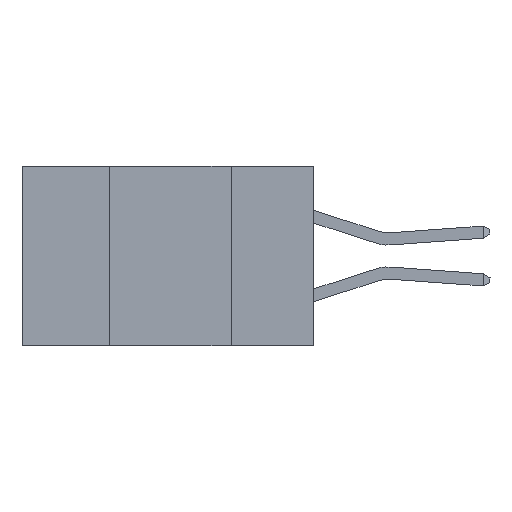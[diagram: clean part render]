
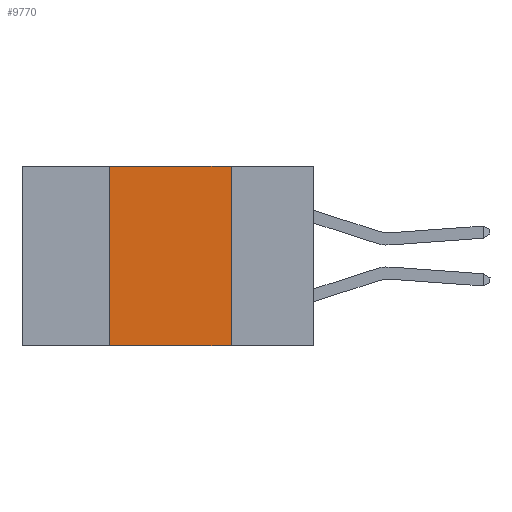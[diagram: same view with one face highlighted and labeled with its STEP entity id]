
A CAD part, left-side view. The second image highlights one B-rep face of the part: STEP entity #9770.
In plain terms, the highlighted planar face has unit normal (-1, 0, 0).
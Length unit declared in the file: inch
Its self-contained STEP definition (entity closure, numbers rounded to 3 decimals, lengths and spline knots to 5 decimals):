
#997 = EDGE_CURVE ( 'NONE', #21251, #8604, #17610, .T. ) ;
#1100 = FACE_OUTER_BOUND ( 'NONE', #4092, .T. ) ;
#1743 = EDGE_CURVE ( 'NONE', #14637, #14149, #7518, .T. ) ;
#2137 = PLANE ( 'NONE',  #11156 ) ;
#4092 = EDGE_LOOP ( 'NONE', ( #19658, #15204, #16624, #13049 ) ) ;
#4861 = CARTESIAN_POINT ( 'NONE',  ( 0., 0.42, 0. ) ) ;
#5753 = DIRECTION ( 'NONE',  ( 1., 0., 0. ) ) ;
#5882 = LINE ( 'NONE', #19341, #19197 ) ;
#6558 = EDGE_CURVE ( 'NONE', #14637, #21251, #21661, .T. ) ;
#7508 = DIRECTION ( 'NONE',  ( 0., -1., 0. ) ) ;
#7518 = LINE ( 'NONE', #14597, #21295 ) ;
#8604 = VERTEX_POINT ( 'NONE', #13218 ) ;
#9770 = ADVANCED_FACE ( 'NONE', ( #1100 ), #2137, .F. ) ;
#10124 = CARTESIAN_POINT ( 'NONE',  ( 0., 0.42, -0.37 ) ) ;
#10190 = EDGE_CURVE ( 'NONE', #8604, #14149, #5882, .T. ) ;
#11156 = AXIS2_PLACEMENT_3D ( 'NONE', #21306, #5753, #17961 ) ;
#12360 = DIRECTION ( 'NONE',  ( 0., 0., 1. ) ) ;
#13049 = ORIENTED_EDGE ( 'NONE', *, *, #1743, .T. ) ;
#13218 = CARTESIAN_POINT ( 'NONE',  ( 0., 0.17, 0. ) ) ;
#14149 = VERTEX_POINT ( 'NONE', #19370 ) ;
#14527 = DIRECTION ( 'NONE',  ( 0., -1., 0. ) ) ;
#14597 = CARTESIAN_POINT ( 'NONE',  ( 0., 0.6, -0.37 ) ) ;
#14637 = VERTEX_POINT ( 'NONE', #10124 ) ;
#15204 = ORIENTED_EDGE ( 'NONE', *, *, #997, .F. ) ;
#16624 = ORIENTED_EDGE ( 'NONE', *, *, #6558, .F. ) ;
#17461 = CARTESIAN_POINT ( 'NONE',  ( 0., 0.42, 0. ) ) ;
#17610 = LINE ( 'NONE', #17735, #22124 ) ;
#17735 = CARTESIAN_POINT ( 'NONE',  ( 0., 0.6, 0. ) ) ;
#17961 = DIRECTION ( 'NONE',  ( 0., 0., -1. ) ) ;
#19197 = VECTOR ( 'NONE', #21068, 39.37008 ) ;
#19341 = CARTESIAN_POINT ( 'NONE',  ( 0., 0.17, 0. ) ) ;
#19370 = CARTESIAN_POINT ( 'NONE',  ( 0., 0.17, -0.37 ) ) ;
#19658 = ORIENTED_EDGE ( 'NONE', *, *, #10190, .F. ) ;
#21068 = DIRECTION ( 'NONE',  ( 0., 0., -1. ) ) ;
#21110 = VECTOR ( 'NONE', #12360, 39.37008 ) ;
#21251 = VERTEX_POINT ( 'NONE', #4861 ) ;
#21295 = VECTOR ( 'NONE', #14527, 39.37008 ) ;
#21306 = CARTESIAN_POINT ( 'NONE',  ( 0., 0.6, 0. ) ) ;
#21661 = LINE ( 'NONE', #17461, #21110 ) ;
#22124 = VECTOR ( 'NONE', #7508, 39.37008 ) ;
